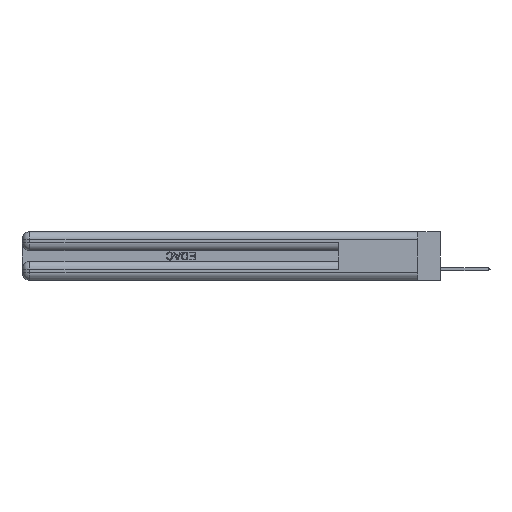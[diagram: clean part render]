
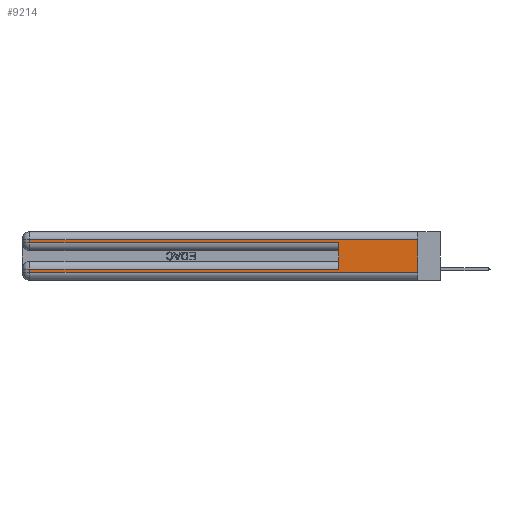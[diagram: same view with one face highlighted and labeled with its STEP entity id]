
A CAD part, left-side view. The second image highlights one B-rep face of the part: STEP entity #9214.
In plain terms, the highlighted planar face has unit normal (-1, 0, 0).
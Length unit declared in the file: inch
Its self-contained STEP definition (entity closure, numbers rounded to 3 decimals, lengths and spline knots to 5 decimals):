
#994 = VERTEX_POINT ( 'NONE', #34823 ) ;
#1483 = CARTESIAN_POINT ( 'NONE',  ( 0., 0., 0.37 ) ) ;
#1941 = CARTESIAN_POINT ( 'NONE',  ( 0., 0., 0.37 ) ) ;
#2085 = VECTOR ( 'NONE', #27318, 39.37008 ) ;
#2477 = DIRECTION ( 'NONE',  ( 0., 0., -1. ) ) ;
#2479 = EDGE_CURVE ( 'NONE', #5544, #22516, #28026, .T. ) ;
#4274 = CARTESIAN_POINT ( 'NONE',  ( 0., 2.94, 0.37 ) ) ;
#4310 = LINE ( 'NONE', #39709, #28298 ) ;
#4498 = VECTOR ( 'NONE', #7559, 39.37008 ) ;
#4565 = ORIENTED_EDGE ( 'NONE', *, *, #24770, .T. ) ;
#4650 = EDGE_CURVE ( 'NONE', #18497, #21669, #8261, .T. ) ;
#5366 = PLANE ( 'NONE',  #17063 ) ;
#5544 = VERTEX_POINT ( 'NONE', #10108 ) ;
#5974 = EDGE_CURVE ( 'NONE', #22516, #44758, #4310, .T. ) ;
#6150 = CARTESIAN_POINT ( 'NONE',  ( 0., 2.94, 0.085 ) ) ;
#6387 = ORIENTED_EDGE ( 'NONE', *, *, #10534, .F. ) ;
#7314 = ORIENTED_EDGE ( 'NONE', *, *, #5974, .T. ) ;
#7559 = DIRECTION ( 'NONE',  ( 0., 0., 1. ) ) ;
#8261 = LINE ( 'NONE', #13482, #2085 ) ;
#9214 = ADVANCED_FACE ( 'NONE', ( #31341 ), #5366, .F. ) ;
#10072 = LINE ( 'NONE', #1941, #44057 ) ;
#10108 = CARTESIAN_POINT ( 'NONE',  ( 0., 2.94, 0.31 ) ) ;
#10534 = EDGE_CURVE ( 'NONE', #31650, #21669, #10072, .T. ) ;
#11096 = VECTOR ( 'NONE', #2477, 39.37008 ) ;
#11779 = CARTESIAN_POINT ( 'NONE',  ( 0., 0.6, 0.145 ) ) ;
#11852 = VECTOR ( 'NONE', #18455, 39.37008 ) ;
#12257 = CARTESIAN_POINT ( 'NONE',  ( 0., 0., 0.06 ) ) ;
#12289 = DIRECTION ( 'NONE',  ( 0., 1., 0. ) ) ;
#13225 = EDGE_CURVE ( 'NONE', #31650, #5544, #24780, .T. ) ;
#13482 = CARTESIAN_POINT ( 'NONE',  ( 0., 0., 0.06 ) ) ;
#14044 = LINE ( 'NONE', #11779, #4498 ) ;
#14445 = VERTEX_POINT ( 'NONE', #6150 ) ;
#15070 = CARTESIAN_POINT ( 'NONE',  ( 0., 0., 0.31 ) ) ;
#15325 = VECTOR ( 'NONE', #12289, 39.37008 ) ;
#15982 = CARTESIAN_POINT ( 'NONE',  ( 0., 0., 0.085 ) ) ;
#16179 = DIRECTION ( 'NONE',  ( 0., 0., -1. ) ) ;
#17063 = AXIS2_PLACEMENT_3D ( 'NONE', #1483, #23181, #40593 ) ;
#18455 = DIRECTION ( 'NONE',  ( 0., 0., -1. ) ) ;
#18497 = VERTEX_POINT ( 'NONE', #40861 ) ;
#18808 = EDGE_CURVE ( 'NONE', #994, #44758, #14044, .T. ) ;
#20959 = VECTOR ( 'NONE', #44784, 39.37008 ) ;
#21669 = VERTEX_POINT ( 'NONE', #12257 ) ;
#22516 = VERTEX_POINT ( 'NONE', #29462 ) ;
#23181 = DIRECTION ( 'NONE',  ( 1., 0., 0. ) ) ;
#24770 = EDGE_CURVE ( 'NONE', #994, #14445, #40425, .T. ) ;
#24780 = LINE ( 'NONE', #15070, #15325 ) ;
#27318 = DIRECTION ( 'NONE',  ( 0., -1., 0. ) ) ;
#28015 = CARTESIAN_POINT ( 'NONE',  ( 0., 0., 0.31 ) ) ;
#28026 = LINE ( 'NONE', #4274, #11852 ) ;
#28057 = ORIENTED_EDGE ( 'NONE', *, *, #29049, .T. ) ;
#28298 = VECTOR ( 'NONE', #36306, 39.37008 ) ;
#29049 = EDGE_CURVE ( 'NONE', #14445, #18497, #38993, .T. ) ;
#29462 = CARTESIAN_POINT ( 'NONE',  ( 0., 2.94, 0.285 ) ) ;
#31341 = FACE_OUTER_BOUND ( 'NONE', #31738, .T. ) ;
#31650 = VERTEX_POINT ( 'NONE', #28015 ) ;
#31738 = EDGE_LOOP ( 'NONE', ( #6387, #33812, #32462, #7314, #42050, #4565, #28057, #40407 ) ) ;
#32462 = ORIENTED_EDGE ( 'NONE', *, *, #2479, .T. ) ;
#32855 = CARTESIAN_POINT ( 'NONE',  ( 0., 0.6, 0.285 ) ) ;
#33812 = ORIENTED_EDGE ( 'NONE', *, *, #13225, .T. ) ;
#34823 = CARTESIAN_POINT ( 'NONE',  ( 0., 0.6, 0.085 ) ) ;
#36306 = DIRECTION ( 'NONE',  ( 0., -1., 0. ) ) ;
#37727 = CARTESIAN_POINT ( 'NONE',  ( 0., 2.94, 0.37 ) ) ;
#38993 = LINE ( 'NONE', #37727, #11096 ) ;
#39709 = CARTESIAN_POINT ( 'NONE',  ( 0., 0., 0.285 ) ) ;
#40407 = ORIENTED_EDGE ( 'NONE', *, *, #4650, .T. ) ;
#40425 = LINE ( 'NONE', #15982, #20959 ) ;
#40593 = DIRECTION ( 'NONE',  ( 0., 0., -1. ) ) ;
#40861 = CARTESIAN_POINT ( 'NONE',  ( 0., 2.94, 0.06 ) ) ;
#42050 = ORIENTED_EDGE ( 'NONE', *, *, #18808, .F. ) ;
#44057 = VECTOR ( 'NONE', #16179, 39.37008 ) ;
#44758 = VERTEX_POINT ( 'NONE', #32855 ) ;
#44784 = DIRECTION ( 'NONE',  ( 0., 1., 0. ) ) ;
